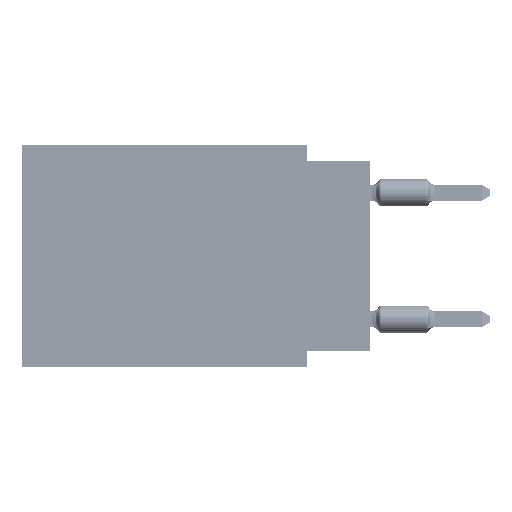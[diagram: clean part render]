
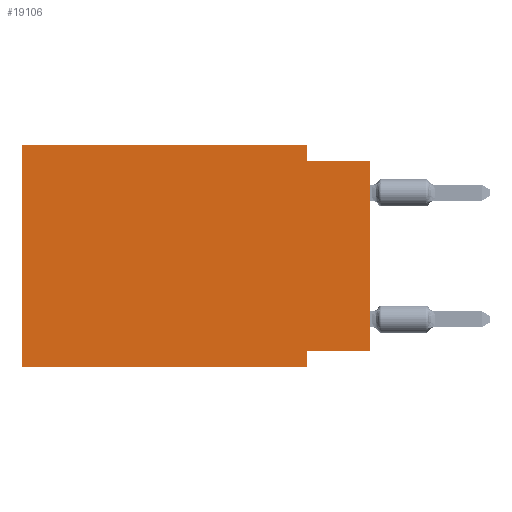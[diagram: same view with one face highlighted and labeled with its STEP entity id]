
A CAD part, left-side view. The second image highlights one B-rep face of the part: STEP entity #19106.
In plain terms, the highlighted planar face has unit normal (-1, 0, 0).
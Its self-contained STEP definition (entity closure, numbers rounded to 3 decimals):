
#174 = LINE ( 'NONE', #557, #60658 ) ;
#557 = CARTESIAN_POINT ( 'NONE',  ( 0., 2.54, 0. ) ) ;
#1918 = EDGE_CURVE ( 'NONE', #54279, #62217, #174, .T. ) ;
#2438 = VERTEX_POINT ( 'NONE', #70180 ) ;
#2540 = DIRECTION ( 'NONE',  ( 0., -1., 0. ) ) ;
#2726 = CARTESIAN_POINT ( 'NONE',  ( 0., 0., -8.255 ) ) ;
#4719 = VECTOR ( 'NONE', #51873, 1000. ) ;
#6133 = FACE_OUTER_BOUND ( 'NONE', #15619, .T. ) ;
#8226 = LINE ( 'NONE', #72613, #12779 ) ;
#9814 = VERTEX_POINT ( 'NONE', #55305 ) ;
#10587 = CARTESIAN_POINT ( 'NONE',  ( 0., 2.54, 0. ) ) ;
#12779 = VECTOR ( 'NONE', #26129, 1000. ) ;
#13399 = LINE ( 'NONE', #2726, #37624 ) ;
#13972 = CARTESIAN_POINT ( 'NONE',  ( 0., 13.97, 0. ) ) ;
#14242 = ORIENTED_EDGE ( 'NONE', *, *, #1918, .F. ) ;
#15463 = CARTESIAN_POINT ( 'NONE',  ( 0., 0., -0.635 ) ) ;
#15619 = EDGE_LOOP ( 'NONE', ( #17415, #55817, #14242, #47326, #20416, #52315, #68802, #36399 ) ) ;
#17026 = DIRECTION ( 'NONE',  ( 0., -1., 0. ) ) ;
#17415 = ORIENTED_EDGE ( 'NONE', *, *, #63411, .T. ) ;
#18540 = VERTEX_POINT ( 'NONE', #40533 ) ;
#19106 = ADVANCED_FACE ( 'NONE', ( #6133 ), #30483, .F. ) ;
#19768 = EDGE_CURVE ( 'NONE', #32634, #35810, #28598, .T. ) ;
#20124 = VECTOR ( 'NONE', #47747, 1000. ) ;
#20416 = ORIENTED_EDGE ( 'NONE', *, *, #19768, .F. ) ;
#21446 = VECTOR ( 'NONE', #72650, 1000. ) ;
#21555 = LINE ( 'NONE', #15463, #21446 ) ;
#24872 = LINE ( 'NONE', #25258, #20124 ) ;
#25258 = CARTESIAN_POINT ( 'NONE',  ( 0., 0., 0. ) ) ;
#25972 = DIRECTION ( 'NONE',  ( 0., 1., 0. ) ) ;
#26129 = DIRECTION ( 'NONE',  ( 0., 0., -1. ) ) ;
#28598 = LINE ( 'NONE', #75089, #4719 ) ;
#30483 = PLANE ( 'NONE',  #65481 ) ;
#32597 = VECTOR ( 'NONE', #17026, 1000. ) ;
#32612 = CARTESIAN_POINT ( 'NONE',  ( 0., 13.97, -8.89 ) ) ;
#32634 = VERTEX_POINT ( 'NONE', #32612 ) ;
#33383 = EDGE_CURVE ( 'NONE', #34375, #2438, #13399, .T. ) ;
#33653 = CARTESIAN_POINT ( 'NONE',  ( 0., 0., -8.255 ) ) ;
#34375 = VERTEX_POINT ( 'NONE', #33653 ) ;
#35810 = VERTEX_POINT ( 'NONE', #42191 ) ;
#36399 = ORIENTED_EDGE ( 'NONE', *, *, #33383, .F. ) ;
#37624 = VECTOR ( 'NONE', #25972, 1000. ) ;
#40533 = CARTESIAN_POINT ( 'NONE',  ( 0., 0., -0.635 ) ) ;
#41556 = CARTESIAN_POINT ( 'NONE',  ( 0., 13.97, 0. ) ) ;
#42191 = CARTESIAN_POINT ( 'NONE',  ( 0., 13.97, 0. ) ) ;
#42318 = DIRECTION ( 'NONE',  ( 1., 0., 0. ) ) ;
#43815 = CARTESIAN_POINT ( 'NONE',  ( 0., 2.54, -0.635 ) ) ;
#46933 = EDGE_CURVE ( 'NONE', #62217, #18540, #21555, .T. ) ;
#47051 = DIRECTION ( 'NONE',  ( 0., 0., -1. ) ) ;
#47326 = ORIENTED_EDGE ( 'NONE', *, *, #70006, .F. ) ;
#47747 = DIRECTION ( 'NONE',  ( 0., 0., 1. ) ) ;
#48988 = EDGE_CURVE ( 'NONE', #32634, #9814, #69217, .T. ) ;
#51784 = EDGE_CURVE ( 'NONE', #2438, #9814, #8226, .T. ) ;
#51873 = DIRECTION ( 'NONE',  ( 0., 0., 1. ) ) ;
#52315 = ORIENTED_EDGE ( 'NONE', *, *, #48988, .T. ) ;
#54279 = VERTEX_POINT ( 'NONE', #10587 ) ;
#55305 = CARTESIAN_POINT ( 'NONE',  ( 0., 2.54, -8.89 ) ) ;
#55817 = ORIENTED_EDGE ( 'NONE', *, *, #46933, .F. ) ;
#56297 = CARTESIAN_POINT ( 'NONE',  ( 0., 13.97, -8.89 ) ) ;
#59183 = VECTOR ( 'NONE', #2540, 1000. ) ;
#60658 = VECTOR ( 'NONE', #47051, 1000. ) ;
#62217 = VERTEX_POINT ( 'NONE', #43815 ) ;
#63411 = EDGE_CURVE ( 'NONE', #34375, #18540, #24872, .T. ) ;
#65166 = DIRECTION ( 'NONE',  ( 0., 0., -1. ) ) ;
#65481 = AXIS2_PLACEMENT_3D ( 'NONE', #41556, #42318, #65166 ) ;
#68802 = ORIENTED_EDGE ( 'NONE', *, *, #51784, .F. ) ;
#69217 = LINE ( 'NONE', #56297, #32597 ) ;
#70006 = EDGE_CURVE ( 'NONE', #35810, #54279, #71888, .T. ) ;
#70180 = CARTESIAN_POINT ( 'NONE',  ( 0., 2.54, -8.255 ) ) ;
#71888 = LINE ( 'NONE', #13972, #59183 ) ;
#72613 = CARTESIAN_POINT ( 'NONE',  ( 0., 2.54, -8.89 ) ) ;
#72650 = DIRECTION ( 'NONE',  ( 0., -1., 0. ) ) ;
#75089 = CARTESIAN_POINT ( 'NONE',  ( 0., 13.97, 0. ) ) ;
